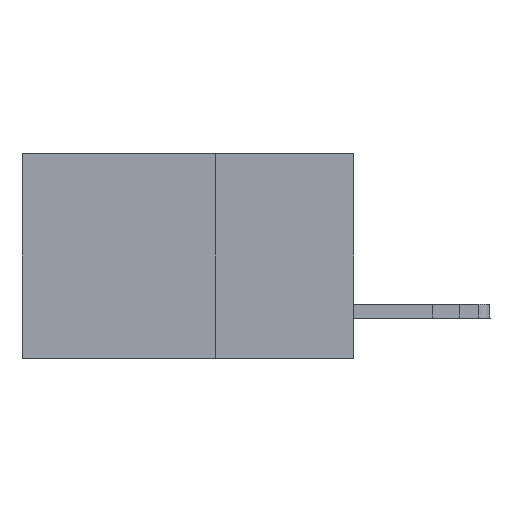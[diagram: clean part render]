
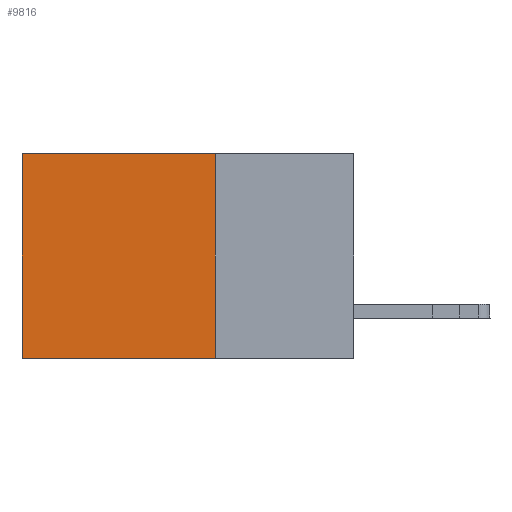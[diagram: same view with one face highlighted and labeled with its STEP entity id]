
A CAD part, left-side view. The second image highlights one B-rep face of the part: STEP entity #9816.
In plain terms, the highlighted planar face has unit normal (-1, 0, 0).
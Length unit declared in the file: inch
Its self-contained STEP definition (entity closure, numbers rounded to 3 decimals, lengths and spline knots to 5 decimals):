
#593 = DIRECTION ( 'NONE',  ( 0., 0., -1. ) ) ;
#631 = DIRECTION ( 'NONE',  ( 0., 1., 0. ) ) ;
#1158 = CARTESIAN_POINT ( 'NONE',  ( 0.2875, 0.25, -0.37 ) ) ;
#1638 = CARTESIAN_POINT ( 'NONE',  ( 0.2875, 0.25, 0. ) ) ;
#1952 = VERTEX_POINT ( 'NONE', #6658 ) ;
#2748 = VECTOR ( 'NONE', #11372, 39.37008 ) ;
#2788 = PLANE ( 'NONE',  #9978 ) ;
#4140 = CARTESIAN_POINT ( 'NONE',  ( 0.2875, 0.25, 0. ) ) ;
#4448 = CARTESIAN_POINT ( 'NONE',  ( 0.2875, 0.25, -0.37 ) ) ;
#4676 = CARTESIAN_POINT ( 'NONE',  ( 0.2875, 0.6, -0.37 ) ) ;
#4891 = FACE_OUTER_BOUND ( 'NONE', #10405, .T. ) ;
#5485 = EDGE_CURVE ( 'NONE', #17541, #15520, #17415, .T. ) ;
#5916 = LINE ( 'NONE', #8860, #10045 ) ;
#6243 = EDGE_CURVE ( 'NONE', #12286, #1952, #5916, .T. ) ;
#6658 = CARTESIAN_POINT ( 'NONE',  ( 0.2875, 0.6, 0. ) ) ;
#6872 = DIRECTION ( 'NONE',  ( 0., 0., -1. ) ) ;
#7545 = ORIENTED_EDGE ( 'NONE', *, *, #10882, .F. ) ;
#8860 = CARTESIAN_POINT ( 'NONE',  ( 0.2875, 0.25, 0. ) ) ;
#9587 = VECTOR ( 'NONE', #16457, 39.37008 ) ;
#9816 = ADVANCED_FACE ( 'NONE', ( #4891 ), #2788, .F. ) ;
#9978 = AXIS2_PLACEMENT_3D ( 'NONE', #4140, #15234, #6872 ) ;
#10045 = VECTOR ( 'NONE', #631, 39.37008 ) ;
#10405 = EDGE_LOOP ( 'NONE', ( #15484, #12934, #7545, #13731 ) ) ;
#10489 = LINE ( 'NONE', #12368, #9587 ) ;
#10882 = EDGE_CURVE ( 'NONE', #12286, #17541, #10489, .T. ) ;
#11372 = DIRECTION ( 'NONE',  ( 0., 1., 0. ) ) ;
#11801 = EDGE_CURVE ( 'NONE', #1952, #15520, #12408, .T. ) ;
#12286 = VERTEX_POINT ( 'NONE', #1638 ) ;
#12368 = CARTESIAN_POINT ( 'NONE',  ( 0.2875, 0.25, 0. ) ) ;
#12408 = LINE ( 'NONE', #14406, #15631 ) ;
#12934 = ORIENTED_EDGE ( 'NONE', *, *, #5485, .F. ) ;
#13731 = ORIENTED_EDGE ( 'NONE', *, *, #6243, .T. ) ;
#14406 = CARTESIAN_POINT ( 'NONE',  ( 0.2875, 0.6, 0. ) ) ;
#15234 = DIRECTION ( 'NONE',  ( 1., 0., 0. ) ) ;
#15484 = ORIENTED_EDGE ( 'NONE', *, *, #11801, .T. ) ;
#15520 = VERTEX_POINT ( 'NONE', #4676 ) ;
#15631 = VECTOR ( 'NONE', #593, 39.37008 ) ;
#16457 = DIRECTION ( 'NONE',  ( 0., 0., -1. ) ) ;
#17415 = LINE ( 'NONE', #4448, #2748 ) ;
#17541 = VERTEX_POINT ( 'NONE', #1158 ) ;
